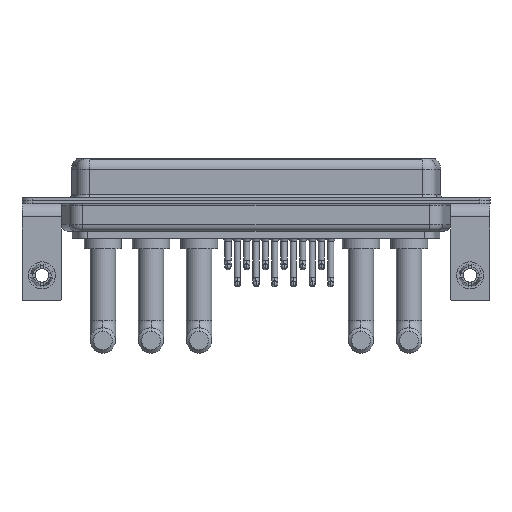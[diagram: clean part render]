
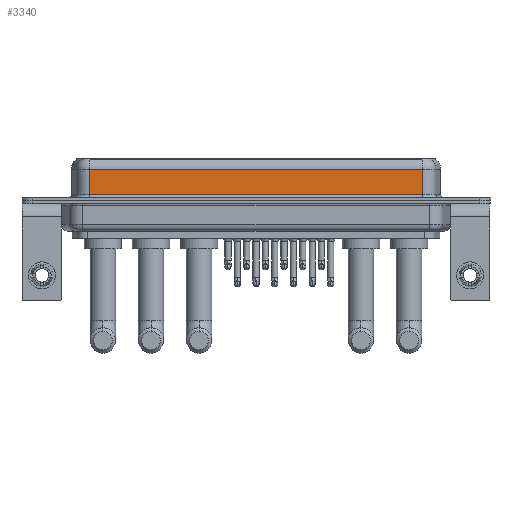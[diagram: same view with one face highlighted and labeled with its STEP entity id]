
A CAD part, front view. The second image highlights one B-rep face of the part: STEP entity #3340.
In plain terms, the highlighted planar face has unit normal (0, -1, 0).
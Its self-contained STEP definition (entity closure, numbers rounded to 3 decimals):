
#174 = LINE ( 'NONE', #18929, #17296 ) ;
#1354 = DIRECTION ( 'NONE',  ( 1., 0., 0. ) ) ;
#1780 = DIRECTION ( 'NONE',  ( 0., 0., -1. ) ) ;
#2060 = ORIENTED_EDGE ( 'NONE', *, *, #21027, .T. ) ;
#3340 = ADVANCED_FACE ( 'NONE', ( #3597 ), #7797, .F. ) ;
#3597 = FACE_OUTER_BOUND ( 'NONE', #17077, .T. ) ;
#3727 = DIRECTION ( 'NONE',  ( -1., 0., 0. ) ) ;
#4778 = LINE ( 'NONE', #20658, #5840 ) ;
#5840 = VECTOR ( 'NONE', #1354, 1000. ) ;
#6000 = VECTOR ( 'NONE', #1780, 1000. ) ;
#7797 = PLANE ( 'NONE',  #8838 ) ;
#8838 = AXIS2_PLACEMENT_3D ( 'NONE', #18182, #12506, #20954 ) ;
#9299 = VERTEX_POINT ( 'NONE', #12167 ) ;
#9556 = CARTESIAN_POINT ( 'NONE',  ( 7.038, -3.95, 4.65 ) ) ;
#9704 = CARTESIAN_POINT ( 'NONE',  ( 56.462, -3.95, 6.4 ) ) ;
#10493 = LINE ( 'NONE', #17445, #6000 ) ;
#10828 = EDGE_CURVE ( 'NONE', #9299, #13303, #14838, .T. ) ;
#12167 = CARTESIAN_POINT ( 'NONE',  ( 56.462, -3.95, 4.65 ) ) ;
#12506 = DIRECTION ( 'NONE',  ( 0., 1., 0. ) ) ;
#13303 = VERTEX_POINT ( 'NONE', #16066 ) ;
#13843 = ORIENTED_EDGE ( 'NONE', *, *, #13974, .T. ) ;
#13974 = EDGE_CURVE ( 'NONE', #21474, #13303, #4778, .T. ) ;
#14838 = LINE ( 'NONE', #9704, #17441 ) ;
#15130 = VERTEX_POINT ( 'NONE', #9556 ) ;
#16066 = CARTESIAN_POINT ( 'NONE',  ( 56.462, -3.95, 0.9 ) ) ;
#17077 = EDGE_LOOP ( 'NONE', ( #21479, #21071, #2060, #13843 ) ) ;
#17296 = VECTOR ( 'NONE', #3727, 1000. ) ;
#17441 = VECTOR ( 'NONE', #21799, 1000. ) ;
#17445 = CARTESIAN_POINT ( 'NONE',  ( 7.038, -3.95, 6.4 ) ) ;
#18182 = CARTESIAN_POINT ( 'NONE',  ( 56.462, -3.95, 6.4 ) ) ;
#18929 = CARTESIAN_POINT ( 'NONE',  ( 56.462, -3.95, 4.65 ) ) ;
#19849 = CARTESIAN_POINT ( 'NONE',  ( 7.038, -3.95, 0.9 ) ) ;
#20658 = CARTESIAN_POINT ( 'NONE',  ( 56.462, -3.95, 0.9 ) ) ;
#20954 = DIRECTION ( 'NONE',  ( 0., 0., 1. ) ) ;
#21027 = EDGE_CURVE ( 'NONE', #15130, #21474, #10493, .T. ) ;
#21071 = ORIENTED_EDGE ( 'NONE', *, *, #21841, .T. ) ;
#21474 = VERTEX_POINT ( 'NONE', #19849 ) ;
#21479 = ORIENTED_EDGE ( 'NONE', *, *, #10828, .F. ) ;
#21799 = DIRECTION ( 'NONE',  ( 0., 0., -1. ) ) ;
#21841 = EDGE_CURVE ( 'NONE', #9299, #15130, #174, .T. ) ;
